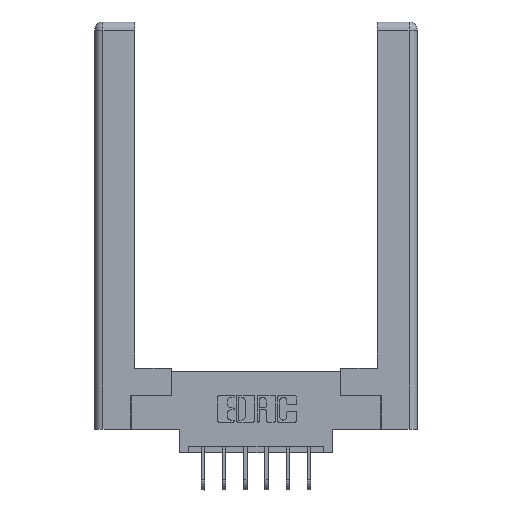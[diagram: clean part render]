
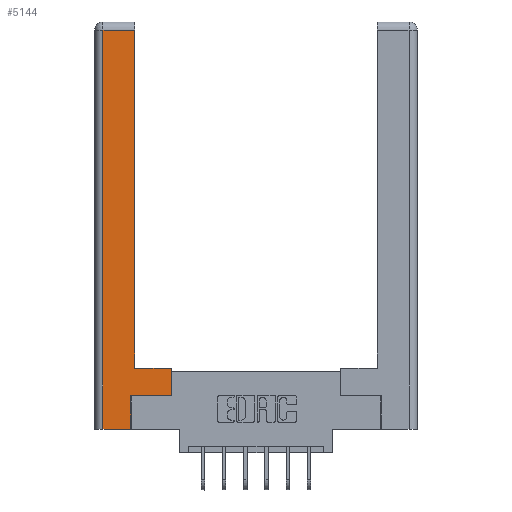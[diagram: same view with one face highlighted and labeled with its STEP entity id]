
A CAD part, top view. The second image highlights one B-rep face of the part: STEP entity #5144.
In plain terms, the highlighted planar face has unit normal (0, 0, 1).
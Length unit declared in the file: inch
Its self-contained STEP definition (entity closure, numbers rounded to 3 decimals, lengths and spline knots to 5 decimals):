
#472 = VECTOR ( 'NONE', #13660, 39.37008 ) ;
#477 = CARTESIAN_POINT ( 'NONE',  ( 0.565, 0.45, 0. ) ) ;
#650 = VECTOR ( 'NONE', #12323, 39.37008 ) ;
#1251 = VERTEX_POINT ( 'NONE', #3078 ) ;
#1374 = VERTEX_POINT ( 'NONE', #3808 ) ;
#1676 = CARTESIAN_POINT ( 'NONE',  ( 0.295, 0.45, 0. ) ) ;
#1848 = VERTEX_POINT ( 'NONE', #6279 ) ;
#2011 = DIRECTION ( 'NONE',  ( 1., 0., 0. ) ) ;
#2018 = EDGE_CURVE ( 'NONE', #1848, #1251, #3189, .T. ) ;
#2389 = EDGE_CURVE ( 'NONE', #7421, #4397, #4685, .T. ) ;
#2483 = LINE ( 'NONE', #9121, #650 ) ;
#2704 = ORIENTED_EDGE ( 'NONE', *, *, #6407, .T. ) ;
#2736 = EDGE_CURVE ( 'NONE', #5780, #4592, #8384, .T. ) ;
#2871 = ORIENTED_EDGE ( 'NONE', *, *, #11919, .T. ) ;
#3078 = CARTESIAN_POINT ( 'NONE',  ( 0.295, 0.45, 0. ) ) ;
#3163 = VECTOR ( 'NONE', #9883, 39.37008 ) ;
#3189 = LINE ( 'NONE', #1676, #8588 ) ;
#3250 = VECTOR ( 'NONE', #7980, 39.37008 ) ;
#3556 = VECTOR ( 'NONE', #13535, 39.37008 ) ;
#3780 = DIRECTION ( 'NONE',  ( -1., 0., 0. ) ) ;
#3808 = CARTESIAN_POINT ( 'NONE',  ( 0.565, 0.245, 0. ) ) ;
#3901 = LINE ( 'NONE', #12551, #3556 ) ;
#4006 = VERTEX_POINT ( 'NONE', #10422 ) ;
#4371 = CARTESIAN_POINT ( 'NONE',  ( 0.0615, 0., 0. ) ) ;
#4397 = VERTEX_POINT ( 'NONE', #13070 ) ;
#4592 = VERTEX_POINT ( 'NONE', #11740 ) ;
#4685 = LINE ( 'NONE', #13559, #6694 ) ;
#4954 = DIRECTION ( 'NONE',  ( -1., 0., 0. ) ) ;
#5144 = ADVANCED_FACE ( 'NONE', ( #12002 ), #9263, .F. ) ;
#5619 = ORIENTED_EDGE ( 'NONE', *, *, #11224, .T. ) ;
#5780 = VERTEX_POINT ( 'NONE', #9235 ) ;
#6110 = ORIENTED_EDGE ( 'NONE', *, *, #2018, .T. ) ;
#6279 = CARTESIAN_POINT ( 'NONE',  ( 0.565, 0.45, 0. ) ) ;
#6407 = EDGE_CURVE ( 'NONE', #1251, #4006, #3901, .T. ) ;
#6694 = VECTOR ( 'NONE', #12536, 39.37008 ) ;
#6989 = LINE ( 'NONE', #477, #472 ) ;
#7223 = ORIENTED_EDGE ( 'NONE', *, *, #2389, .T. ) ;
#7275 = ORIENTED_EDGE ( 'NONE', *, *, #2736, .T. ) ;
#7382 = CARTESIAN_POINT ( 'NONE',  ( 0.265, 0., 0. ) ) ;
#7421 = VERTEX_POINT ( 'NONE', #7382 ) ;
#7628 = VECTOR ( 'NONE', #2011, 39.37008 ) ;
#7778 = EDGE_LOOP ( 'NONE', ( #2704, #13099, #7275, #2871, #7223, #5619, #12309, #6110 ) ) ;
#7980 = DIRECTION ( 'NONE',  ( 1., 0., 0. ) ) ;
#8384 = LINE ( 'NONE', #4371, #3163 ) ;
#8588 = VECTOR ( 'NONE', #3780, 39.37008 ) ;
#8987 = LINE ( 'NONE', #10066, #3250 ) ;
#9121 = CARTESIAN_POINT ( 'NONE',  ( 0.0615, 2.94, 0. ) ) ;
#9193 = AXIS2_PLACEMENT_3D ( 'NONE', #10341, #11423, #4954 ) ;
#9235 = CARTESIAN_POINT ( 'NONE',  ( 0.0615, 2.94, 0. ) ) ;
#9263 = PLANE ( 'NONE',  #9193 ) ;
#9829 = EDGE_CURVE ( 'NONE', #4006, #5780, #2483, .T. ) ;
#9883 = DIRECTION ( 'NONE',  ( 0., -1., 0. ) ) ;
#10066 = CARTESIAN_POINT ( 'NONE',  ( 0.265, 0., 0. ) ) ;
#10177 = LINE ( 'NONE', #12661, #7628 ) ;
#10214 = EDGE_CURVE ( 'NONE', #1374, #1848, #6989, .T. ) ;
#10341 = CARTESIAN_POINT ( 'NONE',  ( 0., 0., 0. ) ) ;
#10422 = CARTESIAN_POINT ( 'NONE',  ( 0.295, 2.94, 0. ) ) ;
#11224 = EDGE_CURVE ( 'NONE', #4397, #1374, #10177, .T. ) ;
#11423 = DIRECTION ( 'NONE',  ( 0., 0., -1. ) ) ;
#11740 = CARTESIAN_POINT ( 'NONE',  ( 0.0615, 0., 0. ) ) ;
#11919 = EDGE_CURVE ( 'NONE', #4592, #7421, #8987, .T. ) ;
#12002 = FACE_OUTER_BOUND ( 'NONE', #7778, .T. ) ;
#12309 = ORIENTED_EDGE ( 'NONE', *, *, #10214, .T. ) ;
#12323 = DIRECTION ( 'NONE',  ( -1., 0., 0. ) ) ;
#12536 = DIRECTION ( 'NONE',  ( 0., 1., 0. ) ) ;
#12551 = CARTESIAN_POINT ( 'NONE',  ( 0.295, 3., 0. ) ) ;
#12661 = CARTESIAN_POINT ( 'NONE',  ( 0.565, 0.245, 0. ) ) ;
#13070 = CARTESIAN_POINT ( 'NONE',  ( 0.265, 0.245, 0. ) ) ;
#13099 = ORIENTED_EDGE ( 'NONE', *, *, #9829, .T. ) ;
#13535 = DIRECTION ( 'NONE',  ( 0., 1., 0. ) ) ;
#13559 = CARTESIAN_POINT ( 'NONE',  ( 0.265, 0.245, 0. ) ) ;
#13660 = DIRECTION ( 'NONE',  ( 0., 1., 0. ) ) ;
